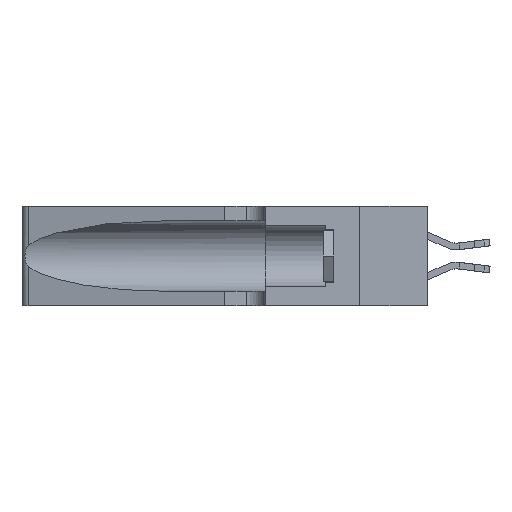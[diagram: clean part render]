
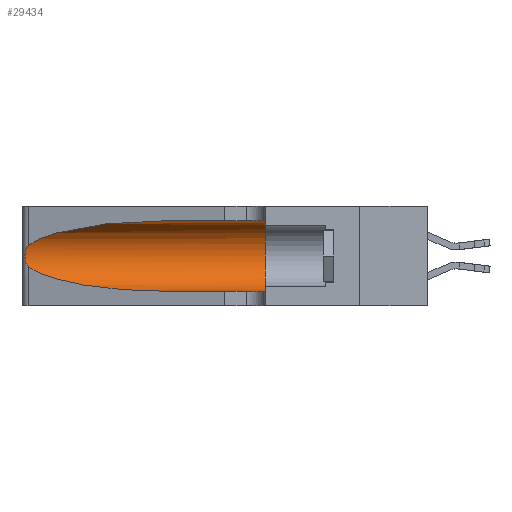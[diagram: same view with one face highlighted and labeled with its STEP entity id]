
A CAD part, left-side view. The second image highlights one B-rep face of the part: STEP entity #29434.
In plain terms, the highlighted cylindrical face has radius 3.308 mm (diameter 6.617 mm), a partial arc.
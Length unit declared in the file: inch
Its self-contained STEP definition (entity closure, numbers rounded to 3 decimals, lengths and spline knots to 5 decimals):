
#247 = CARTESIAN_POINT ( 'NONE',  ( 0.25856, 1.23593, 0.16098 ) ) ;
#364 = EDGE_LOOP ( 'NONE', ( #717, #18388, #6030, #20109, #1591, #10268 ) ) ;
#717 = ORIENTED_EDGE ( 'NONE', *, *, #19794, .T. ) ;
#780 = CARTESIAN_POINT ( 'NONE',  ( 0.1305, 0.72297, 0.05475 ) ) ;
#1027 = EDGE_CURVE ( 'NONE', #27798, #27991, #30484, .T. ) ;
#1206 = VERTEX_POINT ( 'NONE', #26127 ) ;
#1591 = ORIENTED_EDGE ( 'NONE', *, *, #3145, .F. ) ;
#1822 = FACE_OUTER_BOUND ( 'NONE', #364, .T. ) ;
#1827 = VERTEX_POINT ( 'NONE', #7212 ) ;
#2233 = LINE ( 'NONE', #27508, #18330 ) ;
#2522 = CARTESIAN_POINT ( 'NONE',  ( 0.25555, 1.22994, 0.2215 ) ) ;
#2720 = CARTESIAN_POINT ( 'NONE',  ( 0.25487, 1.22718, 0.14631 ) ) ;
#3145 = EDGE_CURVE ( 'NONE', #1827, #27991, #12848, .T. ) ;
#3310 = DIRECTION ( 'NONE',  ( 0., -1., 0. ) ) ;
#4590 = EDGE_CURVE ( 'NONE', #1206, #1827, #2233, .T. ) ;
#5434 = EDGE_CURVE ( 'NONE', #6897, #11217, #24526, .T. ) ;
#6030 = ORIENTED_EDGE ( 'NONE', *, *, #18598, .T. ) ;
#6897 = VERTEX_POINT ( 'NONE', #13105 ) ;
#7212 = CARTESIAN_POINT ( 'NONE',  ( 0.1305, 0.35, 0.31525 ) ) ;
#7322 = CARTESIAN_POINT ( 'NONE',  ( 0.26075, 1.23896, 0.178 ) ) ;
#7413 = DIRECTION ( 'NONE',  ( 0., 1., 0. ) ) ;
#7429 = CARTESIAN_POINT ( 'NONE',  ( 0.25789, 1.23486, 0.15765 ) ) ;
#8208 = CARTESIAN_POINT ( 'NONE',  ( 0.25487, 1.22718, 0.14631 ) ) ;
#10268 = ORIENTED_EDGE ( 'NONE', *, *, #4590, .F. ) ;
#10968 = AXIS2_PLACEMENT_3D ( 'NONE', #18813, #11736, #16639 ) ;
#11217 = VERTEX_POINT ( 'NONE', #23715 ) ;
#11736 = DIRECTION ( 'NONE',  ( 0., -1., 0. ) ) ;
#11797 = VECTOR ( 'NONE', #3310, 39.37008 ) ;
#12263 = CARTESIAN_POINT ( 'NONE',  ( 0.25854, 1.2359, 0.20912 ) ) ;
#12848 = CIRCLE ( 'NONE', #28477, 0.13025 ) ;
#13014 = CARTESIAN_POINT ( 'NONE',  ( 0.2373, 1.15595, 0.08982 ) ) ;
#13105 = CARTESIAN_POINT ( 'NONE',  ( 0.25487, 1.22718, 0.22369 ) ) ;
#14557 = CARTESIAN_POINT ( 'NONE',  ( 0.26075, 1.23896, 0.19203 ) ) ;
#14667 = CARTESIAN_POINT ( 'NONE',  ( 0.26018, 1.23835, 0.19895 ) ) ;
#14775 = CARTESIAN_POINT ( 'NONE',  ( 0.18966, 0.96281, 0.31525 ) ) ;
#16639 = DIRECTION ( 'NONE',  ( 0., 0., -1. ) ) ;
#17068 = CARTESIAN_POINT ( 'NONE',  ( 0.25555, 1.22993, 0.14849 ) ) ;
#17161 = CARTESIAN_POINT ( 'NONE',  ( 0.26017, 1.23833, 0.17102 ) ) ;
#18330 = VECTOR ( 'NONE', #30018, 39.37008 ) ;
#18388 = ORIENTED_EDGE ( 'NONE', *, *, #5434, .T. ) ;
#18598 = EDGE_CURVE ( 'NONE', #11217, #27798, #27814, .T. ) ;
#18813 = CARTESIAN_POINT ( 'NONE',  ( 0.1305, 1.61858, 0.185 ) ) ;
#19244 = CARTESIAN_POINT ( 'NONE',  ( 0.25639, 1.23184, 0.21858 ) ) ;
#19736 = CARTESIAN_POINT ( 'NONE',  ( 0.2373, 1.15595, 0.28018 ) ) ;
#19794 = EDGE_CURVE ( 'NONE', #1206, #6897, #25121, .T. ) ;
#20109 = ORIENTED_EDGE ( 'NONE', *, *, #1027, .T. ) ;
#21614 = CARTESIAN_POINT ( 'NONE',  ( 0.25787, 1.23484, 0.2124 ) ) ;
#21724 = CARTESIAN_POINT ( 'NONE',  ( 0.25487, 1.22718, 0.22369 ) ) ;
#23715 = CARTESIAN_POINT ( 'NONE',  ( 0.25487, 1.22718, 0.14631 ) ) ;
#24108 = DIRECTION ( 'NONE',  ( 0., 0., 1. ) ) ;
#24526 = B_SPLINE_CURVE_WITH_KNOTS ( 'NONE', 3,
 ( #21724, #2522, #19244, #21614, #12263, #14667, #14557, #7322, #17161, #247, #7429, #28953, #17068, #2720 ),
 .UNSPECIFIED., .F., .F.,
 ( 4, 2, 2, 2, 2, 2, 4 ),
 ( 0., 0.00027, 0.00053, 0.00107, 0.0016, 0.00187, 0.00214 ),
 .UNSPECIFIED. ) ;
#24541 = CARTESIAN_POINT ( 'NONE',  ( 0.25487, 1.22718, 0.22369 ) ) ;
#24624 = CARTESIAN_POINT ( 'NONE',  ( 0.1305, 1.61858, 0.05475 ) ) ;
#25121 =( BOUNDED_CURVE ( )  B_SPLINE_CURVE ( 3, ( #27077, #14775, #19736, #24541 ),
 .UNSPECIFIED., .F., .T. ) 
 B_SPLINE_CURVE_WITH_KNOTS ( ( 4, 4 ),
 ( 1.5708, 2.84003 ),
 .UNSPECIFIED. ) 
 CURVE ( )  GEOMETRIC_REPRESENTATION_ITEM ( )  RATIONAL_B_SPLINE_CURVE ( ( 1., 0.87, 0.87, 1. ) ) 
 REPRESENTATION_ITEM ( '' )  );
#25717 = CYLINDRICAL_SURFACE ( 'NONE', #10968, 0.13025 ) ;
#26127 = CARTESIAN_POINT ( 'NONE',  ( 0.1305, 0.72297, 0.31525 ) ) ;
#27077 = CARTESIAN_POINT ( 'NONE',  ( 0.1305, 0.72297, 0.31525 ) ) ;
#27091 = CARTESIAN_POINT ( 'NONE',  ( 0.18966, 0.96281, 0.05475 ) ) ;
#27508 = CARTESIAN_POINT ( 'NONE',  ( 0.1305, 1.61858, 0.31525 ) ) ;
#27798 = VERTEX_POINT ( 'NONE', #28075 ) ;
#27814 =( BOUNDED_CURVE ( )  B_SPLINE_CURVE ( 3, ( #8208, #13014, #27091, #780 ),
 .UNSPECIFIED., .F., .F. ) 
 B_SPLINE_CURVE_WITH_KNOTS ( ( 4, 4 ),
 ( 3.44316, 4.71239 ),
 .UNSPECIFIED. ) 
 CURVE ( )  GEOMETRIC_REPRESENTATION_ITEM ( )  RATIONAL_B_SPLINE_CURVE ( ( 1., 0.87, 0.87, 1. ) ) 
 REPRESENTATION_ITEM ( '' )  );
#27991 = VERTEX_POINT ( 'NONE', #28181 ) ;
#28075 = CARTESIAN_POINT ( 'NONE',  ( 0.1305, 0.72297, 0.05475 ) ) ;
#28181 = CARTESIAN_POINT ( 'NONE',  ( 0.1305, 0.35, 0.05475 ) ) ;
#28477 = AXIS2_PLACEMENT_3D ( 'NONE', #28931, #7413, #24108 ) ;
#28931 = CARTESIAN_POINT ( 'NONE',  ( 0.1305, 0.35, 0.185 ) ) ;
#28953 = CARTESIAN_POINT ( 'NONE',  ( 0.25639, 1.23186, 0.15144 ) ) ;
#29434 = ADVANCED_FACE ( 'NONE', ( #1822 ), #25717, .F. ) ;
#30018 = DIRECTION ( 'NONE',  ( 0., -1., 0. ) ) ;
#30484 = LINE ( 'NONE', #24624, #11797 ) ;
